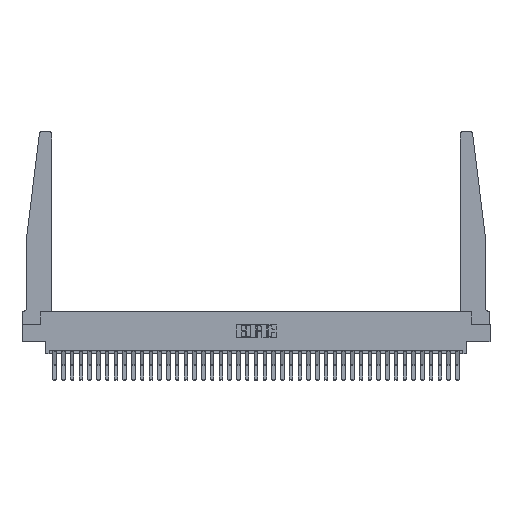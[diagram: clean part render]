
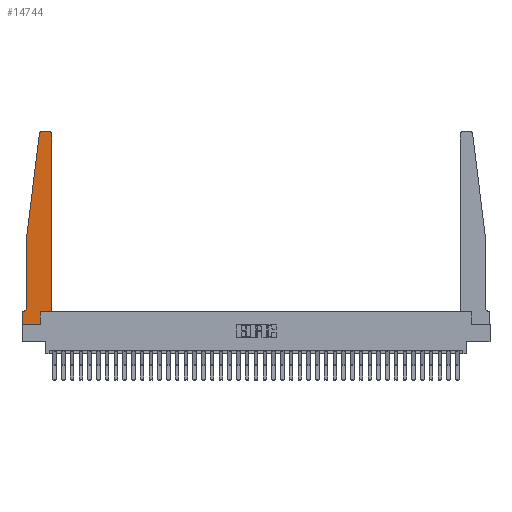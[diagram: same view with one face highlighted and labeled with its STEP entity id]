
A CAD part, top view. The second image highlights one B-rep face of the part: STEP entity #14744.
In plain terms, the highlighted planar face has unit normal (0, 0, 1).
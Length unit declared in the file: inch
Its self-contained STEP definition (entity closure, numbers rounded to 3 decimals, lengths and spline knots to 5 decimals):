
#82 = ORIENTED_EDGE ( 'NONE', *, *, #30138, .T. ) ;
#243 = CARTESIAN_POINT ( 'NONE',  ( 0., 0., 0.37 ) ) ;
#595 = DIRECTION ( 'NONE',  ( -1., 0., 0. ) ) ;
#679 = CARTESIAN_POINT ( 'NONE',  ( 0., 0.1875, 0.37 ) ) ;
#1717 = VECTOR ( 'NONE', #18134, 39.37008 ) ;
#2208 = EDGE_CURVE ( 'NONE', #15684, #23150, #14499, .T. ) ;
#2226 = DIRECTION ( 'NONE',  ( 1., 0., 0. ) ) ;
#2301 = VERTEX_POINT ( 'NONE', #18256 ) ;
#2303 = ORIENTED_EDGE ( 'NONE', *, *, #23827, .T. ) ;
#2537 = CARTESIAN_POINT ( 'NONE',  ( 0.2605, 0., 0.37 ) ) ;
#2729 = CARTESIAN_POINT ( 'NONE',  ( 0.425, 2.72, 0.37 ) ) ;
#3007 = DIRECTION ( 'NONE',  ( 0., 1., 0. ) ) ;
#3073 = DIRECTION ( 'NONE',  ( 0., -1., 0. ) ) ;
#3182 = VERTEX_POINT ( 'NONE', #14896 ) ;
#3186 = LINE ( 'NONE', #8397, #23726 ) ;
#3597 = EDGE_CURVE ( 'NONE', #7513, #33938, #6990, .T. ) ;
#4494 = DIRECTION ( 'NONE',  ( 1., 0., 0. ) ) ;
#4758 = CARTESIAN_POINT ( 'NONE',  ( 0.27653, 2.72, 0.37 ) ) ;
#5031 = LINE ( 'NONE', #34803, #1717 ) ;
#5166 = CARTESIAN_POINT ( 'NONE',  ( 0.015, 0.2375, 0.37 ) ) ;
#5421 = VECTOR ( 'NONE', #13256, 39.37008 ) ;
#6104 = ORIENTED_EDGE ( 'NONE', *, *, #24561, .T. ) ;
#6466 = CARTESIAN_POINT ( 'NONE',  ( 0.24675, 2.72367, 0.37 ) ) ;
#6923 = AXIS2_PLACEMENT_3D ( 'NONE', #4758, #34705, #18567 ) ;
#6990 = LINE ( 'NONE', #33887, #16426 ) ;
#7046 = VERTEX_POINT ( 'NONE', #32614 ) ;
#7227 = CIRCLE ( 'NONE', #27823, 0.05 ) ;
#7277 = CIRCLE ( 'NONE', #30170, 0.03 ) ;
#7513 = VERTEX_POINT ( 'NONE', #2537 ) ;
#7589 = CARTESIAN_POINT ( 'NONE',  ( 0.2605, 0.18, 0.37 ) ) ;
#8397 = CARTESIAN_POINT ( 'NONE',  ( 0.425, 0.18, 0.37 ) ) ;
#9094 = EDGE_CURVE ( 'NONE', #12487, #21895, #7277, .T. ) ;
#9407 = CARTESIAN_POINT ( 'NONE',  ( 0.065, 1.25, 0.37 ) ) ;
#9682 = EDGE_CURVE ( 'NONE', #3182, #22656, #7227, .T. ) ;
#10307 = EDGE_CURVE ( 'NONE', #23150, #3182, #34148, .T. ) ;
#12174 = ORIENTED_EDGE ( 'NONE', *, *, #24306, .T. ) ;
#12423 = CARTESIAN_POINT ( 'NONE',  ( 0.395, 2.75, 0.37 ) ) ;
#12487 = VERTEX_POINT ( 'NONE', #2729 ) ;
#12890 = ORIENTED_EDGE ( 'NONE', *, *, #22115, .T. ) ;
#12918 = ORIENTED_EDGE ( 'NONE', *, *, #9682, .T. ) ;
#12999 = CARTESIAN_POINT ( 'NONE',  ( 0., 0.1875, 0.37 ) ) ;
#13256 = DIRECTION ( 'NONE',  ( 1., 0., 0. ) ) ;
#13884 = LINE ( 'NONE', #243, #29812 ) ;
#14345 = AXIS2_PLACEMENT_3D ( 'NONE', #679, #30098, #19340 ) ;
#14499 = LINE ( 'NONE', #33506, #28360 ) ;
#14744 = ADVANCED_FACE ( 'NONE', ( #27948 ), #22022, .T. ) ;
#14781 = DIRECTION ( 'NONE',  ( 0., -1., 0. ) ) ;
#14896 = CARTESIAN_POINT ( 'NONE',  ( 0.065, 0.2375, 0.37 ) ) ;
#15684 = VERTEX_POINT ( 'NONE', #6466 ) ;
#16059 = ORIENTED_EDGE ( 'NONE', *, *, #9094, .T. ) ;
#16426 = VECTOR ( 'NONE', #20425, 39.37008 ) ;
#16653 = CIRCLE ( 'NONE', #6923, 0.03 ) ;
#17658 = LINE ( 'NONE', #29931, #5421 ) ;
#17907 = DIRECTION ( 'NONE',  ( -0.122, -0.992, 0. ) ) ;
#18134 = DIRECTION ( 'NONE',  ( -1., 0., 0. ) ) ;
#18256 = CARTESIAN_POINT ( 'NONE',  ( 0., 0., 0.37 ) ) ;
#18567 = DIRECTION ( 'NONE',  ( 1., 0., 0. ) ) ;
#19340 = DIRECTION ( 'NONE',  ( 1., 0., 0. ) ) ;
#19374 = VERTEX_POINT ( 'NONE', #12999 ) ;
#19688 = VECTOR ( 'NONE', #3073, 39.37008 ) ;
#19996 = CARTESIAN_POINT ( 'NONE',  ( 0.015, 0.1875, 0.37 ) ) ;
#20425 = DIRECTION ( 'NONE',  ( 0., 1., 0. ) ) ;
#20945 = DIRECTION ( 'NONE',  ( 0., 0., -1. ) ) ;
#21895 = VERTEX_POINT ( 'NONE', #12423 ) ;
#21928 = EDGE_LOOP ( 'NONE', ( #27595, #12174, #32971, #22452, #12918, #23596, #82, #6104, #26279, #2303, #12890, #16059 ) ) ;
#22022 = PLANE ( 'NONE',  #14345 ) ;
#22115 = EDGE_CURVE ( 'NONE', #7046, #12487, #3186, .T. ) ;
#22452 = ORIENTED_EDGE ( 'NONE', *, *, #10307, .T. ) ;
#22656 = VERTEX_POINT ( 'NONE', #19996 ) ;
#23101 = CARTESIAN_POINT ( 'NONE',  ( 0.27653, 2.75, 0.37 ) ) ;
#23150 = VERTEX_POINT ( 'NONE', #34131 ) ;
#23596 = ORIENTED_EDGE ( 'NONE', *, *, #33532, .T. ) ;
#23726 = VECTOR ( 'NONE', #3007, 39.37008 ) ;
#23827 = EDGE_CURVE ( 'NONE', #33938, #7046, #17658, .T. ) ;
#24306 = EDGE_CURVE ( 'NONE', #30705, #15684, #16653, .T. ) ;
#24561 = EDGE_CURVE ( 'NONE', #2301, #7513, #13884, .T. ) ;
#26018 = DIRECTION ( 'NONE',  ( 0., 0., 1. ) ) ;
#26279 = ORIENTED_EDGE ( 'NONE', *, *, #3597, .T. ) ;
#27466 = CARTESIAN_POINT ( 'NONE',  ( 0., 0., 0.37 ) ) ;
#27508 = CARTESIAN_POINT ( 'NONE',  ( 0.065, 0.1875, 0.37 ) ) ;
#27595 = ORIENTED_EDGE ( 'NONE', *, *, #31699, .T. ) ;
#27823 = AXIS2_PLACEMENT_3D ( 'NONE', #5166, #20945, #31897 ) ;
#27867 = LINE ( 'NONE', #27508, #32735 ) ;
#27948 = FACE_OUTER_BOUND ( 'NONE', #21928, .T. ) ;
#28360 = VECTOR ( 'NONE', #17907, 39.37008 ) ;
#29063 = CARTESIAN_POINT ( 'NONE',  ( 0.395, 2.72, 0.37 ) ) ;
#29812 = VECTOR ( 'NONE', #2226, 39.37008 ) ;
#29931 = CARTESIAN_POINT ( 'NONE',  ( 0.425, 0.18, 0.37 ) ) ;
#30098 = DIRECTION ( 'NONE',  ( 0., 0., 1. ) ) ;
#30138 = EDGE_CURVE ( 'NONE', #19374, #2301, #30337, .T. ) ;
#30170 = AXIS2_PLACEMENT_3D ( 'NONE', #29063, #26018, #4494 ) ;
#30337 = LINE ( 'NONE', #27466, #19688 ) ;
#30705 = VERTEX_POINT ( 'NONE', #23101 ) ;
#31699 = EDGE_CURVE ( 'NONE', #21895, #30705, #5031, .T. ) ;
#31897 = DIRECTION ( 'NONE',  ( -1., 0., 0. ) ) ;
#32614 = CARTESIAN_POINT ( 'NONE',  ( 0.425, 0.18, 0.37 ) ) ;
#32647 = VECTOR ( 'NONE', #14781, 39.37008 ) ;
#32735 = VECTOR ( 'NONE', #595, 39.37008 ) ;
#32971 = ORIENTED_EDGE ( 'NONE', *, *, #2208, .T. ) ;
#33506 = CARTESIAN_POINT ( 'NONE',  ( 0.065, 1.25, 0.37 ) ) ;
#33532 = EDGE_CURVE ( 'NONE', #22656, #19374, #27867, .T. ) ;
#33887 = CARTESIAN_POINT ( 'NONE',  ( 0.2605, 0.18, 0.37 ) ) ;
#33938 = VERTEX_POINT ( 'NONE', #7589 ) ;
#34131 = CARTESIAN_POINT ( 'NONE',  ( 0.065, 1.25, 0.37 ) ) ;
#34148 = LINE ( 'NONE', #9407, #32647 ) ;
#34705 = DIRECTION ( 'NONE',  ( 0., 0., 1. ) ) ;
#34803 = CARTESIAN_POINT ( 'NONE',  ( 0.25, 2.75, 0.37 ) ) ;
